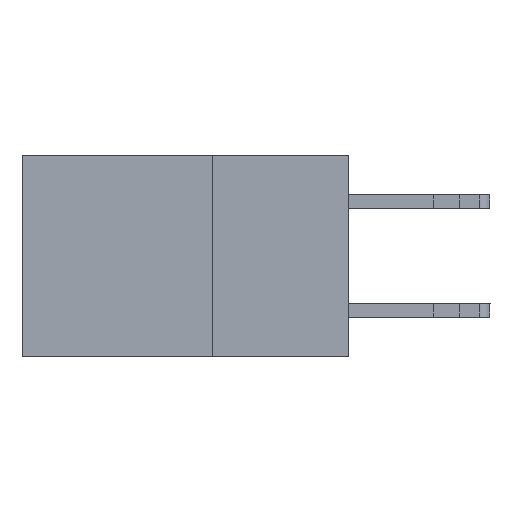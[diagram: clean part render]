
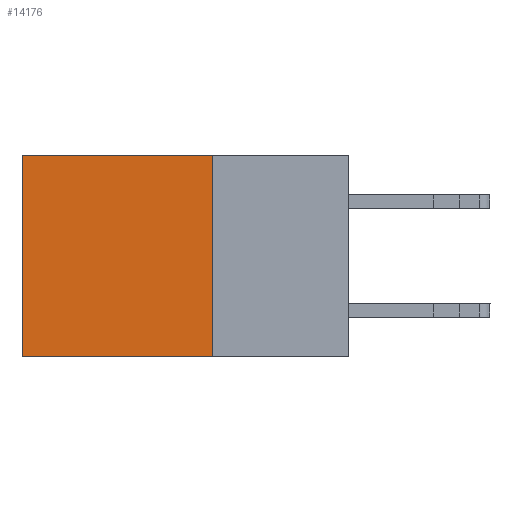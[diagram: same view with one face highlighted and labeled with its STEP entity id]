
A CAD part, left-side view. The second image highlights one B-rep face of the part: STEP entity #14176.
In plain terms, the highlighted planar face has unit normal (-1, 0, 0).
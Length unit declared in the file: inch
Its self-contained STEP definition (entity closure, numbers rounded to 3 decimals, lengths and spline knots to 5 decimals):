
#497 = ORIENTED_EDGE ( 'NONE', *, *, #5004, .F. ) ;
#674 = DIRECTION ( 'NONE',  ( 1., 0., 0. ) ) ;
#1235 = CARTESIAN_POINT ( 'NONE',  ( 0.2615, 0.25, -0.37 ) ) ;
#1408 = AXIS2_PLACEMENT_3D ( 'NONE', #17977, #674, #10913 ) ;
#1435 = LINE ( 'NONE', #10406, #12542 ) ;
#3098 = VECTOR ( 'NONE', #5480, 39.37008 ) ;
#3958 = VECTOR ( 'NONE', #12211, 39.37008 ) ;
#3982 = CARTESIAN_POINT ( 'NONE',  ( 0.2615, 0.25, 0. ) ) ;
#4951 = ORIENTED_EDGE ( 'NONE', *, *, #13637, .T. ) ;
#5004 = EDGE_CURVE ( 'NONE', #11953, #8925, #15770, .T. ) ;
#5480 = DIRECTION ( 'NONE',  ( 0., 1., 0. ) ) ;
#6047 = VERTEX_POINT ( 'NONE', #9084 ) ;
#6191 = CARTESIAN_POINT ( 'NONE',  ( 0.2615, 0.25, 0. ) ) ;
#7456 = EDGE_CURVE ( 'NONE', #6047, #10194, #1435, .T. ) ;
#7830 = LINE ( 'NONE', #10817, #3958 ) ;
#8925 = VERTEX_POINT ( 'NONE', #1235 ) ;
#9055 = EDGE_LOOP ( 'NONE', ( #18361, #15029, #497, #4951 ) ) ;
#9084 = CARTESIAN_POINT ( 'NONE',  ( 0.2615, 0.6, 0. ) ) ;
#10194 = VERTEX_POINT ( 'NONE', #11139 ) ;
#10406 = CARTESIAN_POINT ( 'NONE',  ( 0.2615, 0.6, -0.37 ) ) ;
#10410 = DIRECTION ( 'NONE',  ( 0., 0., -1. ) ) ;
#10817 = CARTESIAN_POINT ( 'NONE',  ( 0.2615, 0.25, -0.37 ) ) ;
#10913 = DIRECTION ( 'NONE',  ( 0., 0., -1. ) ) ;
#11139 = CARTESIAN_POINT ( 'NONE',  ( 0.2615, 0.6, -0.37 ) ) ;
#11237 = LINE ( 'NONE', #3982, #3098 ) ;
#11953 = VERTEX_POINT ( 'NONE', #6191 ) ;
#12211 = DIRECTION ( 'NONE',  ( 0., 1., 0. ) ) ;
#12542 = VECTOR ( 'NONE', #10410, 39.37008 ) ;
#12765 = FACE_OUTER_BOUND ( 'NONE', #9055, .T. ) ;
#13637 = EDGE_CURVE ( 'NONE', #11953, #6047, #11237, .T. ) ;
#14176 = ADVANCED_FACE ( 'NONE', ( #12765 ), #16495, .F. ) ;
#14640 = DIRECTION ( 'NONE',  ( 0., 0., -1. ) ) ;
#14975 = CARTESIAN_POINT ( 'NONE',  ( 0.2615, 0.25, -0.37 ) ) ;
#15029 = ORIENTED_EDGE ( 'NONE', *, *, #15614, .F. ) ;
#15308 = VECTOR ( 'NONE', #14640, 39.37008 ) ;
#15614 = EDGE_CURVE ( 'NONE', #8925, #10194, #7830, .T. ) ;
#15770 = LINE ( 'NONE', #14975, #15308 ) ;
#16495 = PLANE ( 'NONE',  #1408 ) ;
#17977 = CARTESIAN_POINT ( 'NONE',  ( 0.2615, 0.25, -0.37 ) ) ;
#18361 = ORIENTED_EDGE ( 'NONE', *, *, #7456, .T. ) ;
